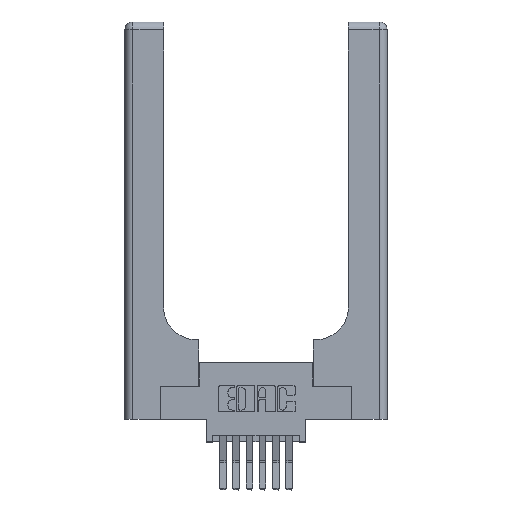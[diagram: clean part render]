
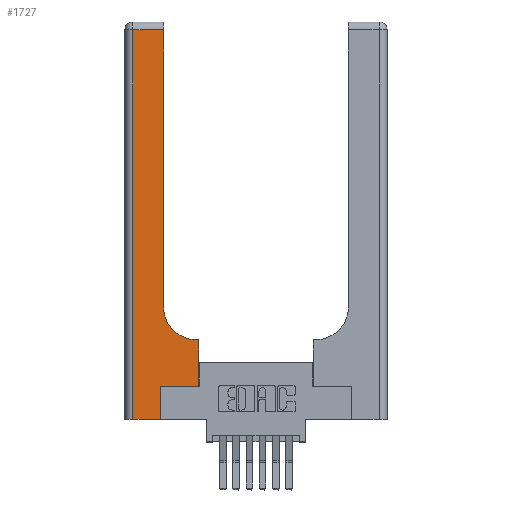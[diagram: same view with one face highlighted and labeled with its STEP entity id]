
A CAD part, top view. The second image highlights one B-rep face of the part: STEP entity #1727.
In plain terms, the highlighted planar face has unit normal (0, 0, 1).
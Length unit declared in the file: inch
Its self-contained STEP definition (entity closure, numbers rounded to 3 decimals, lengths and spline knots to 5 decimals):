
#117 = DIRECTION ( 'NONE',  ( 0., 1., 0. ) ) ;
#372 = AXIS2_PLACEMENT_3D ( 'NONE', #9179, #9083, #8938 ) ;
#1009 = EDGE_LOOP ( 'NONE', ( #5187, #1908, #6188, #14046, #6622, #6945, #6254, #1044, #6683 ) ) ;
#1044 = ORIENTED_EDGE ( 'NONE', *, *, #5489, .T. ) ;
#1329 = VECTOR ( 'NONE', #13399, 39.37008 ) ;
#1621 = DIRECTION ( 'NONE',  ( 0., 1., 0. ) ) ;
#1727 = ADVANCED_FACE ( 'NONE', ( #9050 ), #9222, .F. ) ;
#1819 = EDGE_CURVE ( 'NONE', #2321, #8319, #7607, .T. ) ;
#1856 = CARTESIAN_POINT ( 'NONE',  ( 0., 2.94, 0.37 ) ) ;
#1908 = ORIENTED_EDGE ( 'NONE', *, *, #5092, .T. ) ;
#2321 = VERTEX_POINT ( 'NONE', #4253 ) ;
#2914 = DIRECTION ( 'NONE',  ( 0., 0., -1. ) ) ;
#2944 = CARTESIAN_POINT ( 'NONE',  ( 0.2915, 2.94, 0.37 ) ) ;
#3002 = CARTESIAN_POINT ( 'NONE',  ( 0.269, 0., 0.37 ) ) ;
#3053 = CARTESIAN_POINT ( 'NONE',  ( 0.2915, 0.6, 0.37 ) ) ;
#3372 = LINE ( 'NONE', #6536, #9138 ) ;
#3775 = VERTEX_POINT ( 'NONE', #2944 ) ;
#3894 = DIRECTION ( 'NONE',  ( 0., 1., 0. ) ) ;
#4220 = DIRECTION ( 'NONE',  ( 1., 0., 0. ) ) ;
#4253 = CARTESIAN_POINT ( 'NONE',  ( 0.269, 0.25, 0.37 ) ) ;
#4410 = LINE ( 'NONE', #1856, #1329 ) ;
#4499 = VERTEX_POINT ( 'NONE', #5609 ) ;
#4590 = CARTESIAN_POINT ( 'NONE',  ( 0.5585, 0.6, 0.37 ) ) ;
#4707 = CARTESIAN_POINT ( 'NONE',  ( 0.269, 0.25, 0.37 ) ) ;
#4719 = CARTESIAN_POINT ( 'NONE',  ( 0.2915, 3., 0.37 ) ) ;
#4887 = DIRECTION ( 'NONE',  ( 1., 0., 0. ) ) ;
#5013 = CARTESIAN_POINT ( 'NONE',  ( 0.269, 0., 0.37 ) ) ;
#5092 = EDGE_CURVE ( 'NONE', #3775, #13969, #4410, .T. ) ;
#5097 = LINE ( 'NONE', #7365, #13544 ) ;
#5187 = ORIENTED_EDGE ( 'NONE', *, *, #12495, .T. ) ;
#5330 = VERTEX_POINT ( 'NONE', #12861 ) ;
#5350 = CARTESIAN_POINT ( 'NONE',  ( 0.5415, 0.6, 0.37 ) ) ;
#5489 = EDGE_CURVE ( 'NONE', #5714, #7795, #9637, .T. ) ;
#5609 = CARTESIAN_POINT ( 'NONE',  ( 0.06, 0., 0.37 ) ) ;
#5714 = VERTEX_POINT ( 'NONE', #4590 ) ;
#6187 = LINE ( 'NONE', #12247, #8529 ) ;
#6188 = ORIENTED_EDGE ( 'NONE', *, *, #6534, .T. ) ;
#6254 = ORIENTED_EDGE ( 'NONE', *, *, #7106, .T. ) ;
#6440 = EDGE_CURVE ( 'NONE', #7795, #5330, #9609, .T. ) ;
#6447 = DIRECTION ( 'NONE',  ( 0., -1., 0. ) ) ;
#6450 = CARTESIAN_POINT ( 'NONE',  ( 0.06, 2.94, 0.37 ) ) ;
#6530 = DIRECTION ( 'NONE',  ( -1., 0., 0. ) ) ;
#6534 = EDGE_CURVE ( 'NONE', #13969, #4499, #6187, .T. ) ;
#6536 = CARTESIAN_POINT ( 'NONE',  ( 0., 0., 0.37 ) ) ;
#6571 = VECTOR ( 'NONE', #6530, 39.37008 ) ;
#6622 = ORIENTED_EDGE ( 'NONE', *, *, #10435, .T. ) ;
#6683 = ORIENTED_EDGE ( 'NONE', *, *, #6440, .T. ) ;
#6945 = ORIENTED_EDGE ( 'NONE', *, *, #1819, .T. ) ;
#7106 = EDGE_CURVE ( 'NONE', #8319, #5714, #5097, .T. ) ;
#7365 = CARTESIAN_POINT ( 'NONE',  ( 0.5585, 0.25, 0.37 ) ) ;
#7607 = LINE ( 'NONE', #4707, #13378 ) ;
#7795 = VERTEX_POINT ( 'NONE', #5350 ) ;
#8319 = VERTEX_POINT ( 'NONE', #13115 ) ;
#8529 = VECTOR ( 'NONE', #6447, 39.37008 ) ;
#8938 = DIRECTION ( 'NONE',  ( -1., 0., 0. ) ) ;
#9050 = FACE_OUTER_BOUND ( 'NONE', #1009, .T. ) ;
#9083 = DIRECTION ( 'NONE',  ( 0., 0., -1. ) ) ;
#9138 = VECTOR ( 'NONE', #4220, 39.37008 ) ;
#9179 = CARTESIAN_POINT ( 'NONE',  ( 0., 3., 0.37 ) ) ;
#9222 = PLANE ( 'NONE',  #372 ) ;
#9363 = VECTOR ( 'NONE', #117, 39.37008 ) ;
#9609 = CIRCLE ( 'NONE', #11675, 0.25 ) ;
#9637 = LINE ( 'NONE', #3053, #6571 ) ;
#9833 = CARTESIAN_POINT ( 'NONE',  ( 0.5415, 0.85, 0.37 ) ) ;
#10435 = EDGE_CURVE ( 'NONE', #11581, #2321, #11600, .T. ) ;
#11000 = DIRECTION ( 'NONE',  ( 1., 0., 0. ) ) ;
#11581 = VERTEX_POINT ( 'NONE', #3002 ) ;
#11600 = LINE ( 'NONE', #5013, #14664 ) ;
#11675 = AXIS2_PLACEMENT_3D ( 'NONE', #9833, #2914, #11000 ) ;
#12247 = CARTESIAN_POINT ( 'NONE',  ( 0.06, 3., 0.37 ) ) ;
#12425 = LINE ( 'NONE', #4719, #9363 ) ;
#12495 = EDGE_CURVE ( 'NONE', #5330, #3775, #12425, .T. ) ;
#12861 = CARTESIAN_POINT ( 'NONE',  ( 0.2915, 0.85, 0.37 ) ) ;
#13115 = CARTESIAN_POINT ( 'NONE',  ( 0.5585, 0.25, 0.37 ) ) ;
#13378 = VECTOR ( 'NONE', #4887, 39.37008 ) ;
#13399 = DIRECTION ( 'NONE',  ( -1., 0., 0. ) ) ;
#13544 = VECTOR ( 'NONE', #1621, 39.37008 ) ;
#13969 = VERTEX_POINT ( 'NONE', #6450 ) ;
#14046 = ORIENTED_EDGE ( 'NONE', *, *, #14637, .T. ) ;
#14637 = EDGE_CURVE ( 'NONE', #4499, #11581, #3372, .T. ) ;
#14664 = VECTOR ( 'NONE', #3894, 39.37008 ) ;
